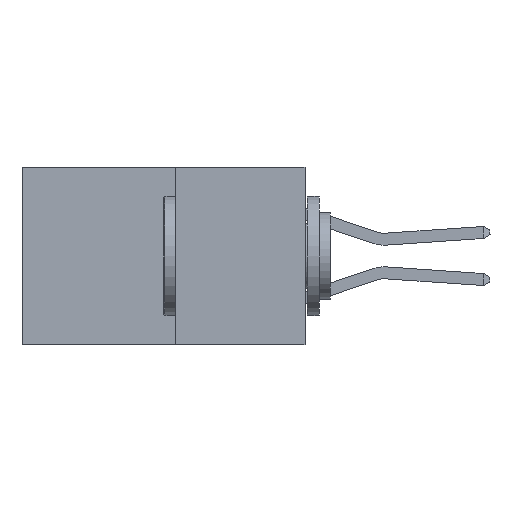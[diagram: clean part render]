
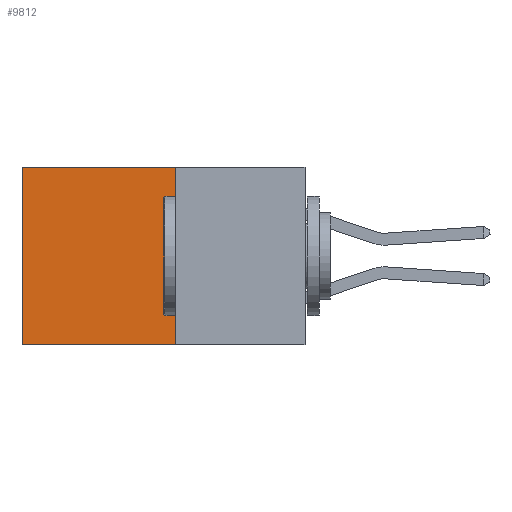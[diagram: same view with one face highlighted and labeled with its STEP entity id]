
A CAD part, left-side view. The second image highlights one B-rep face of the part: STEP entity #9812.
In plain terms, the highlighted planar face has unit normal (-1, 0, 0).
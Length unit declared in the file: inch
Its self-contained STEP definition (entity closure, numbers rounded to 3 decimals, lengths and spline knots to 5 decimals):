
#578 = EDGE_CURVE ( 'NONE', #14383, #9745, #9992, .T. ) ;
#730 = DIRECTION ( 'NONE',  ( 0., 0., -1. ) ) ;
#804 = DIRECTION ( 'NONE',  ( 0., 1., 0. ) ) ;
#988 = CARTESIAN_POINT ( 'NONE',  ( 0.277, 0.27, -0.37 ) ) ;
#1501 = VECTOR ( 'NONE', #804, 39.37008 ) ;
#1978 = CARTESIAN_POINT ( 'NONE',  ( 0.277, 0.59, -0.37 ) ) ;
#2117 = LINE ( 'NONE', #7203, #9323 ) ;
#2404 = ORIENTED_EDGE ( 'NONE', *, *, #6693, .T. ) ;
#3369 = AXIS2_PLACEMENT_3D ( 'NONE', #15497, #8849, #730 ) ;
#3455 = CARTESIAN_POINT ( 'NONE',  ( 0.277, 0.27, -0.37 ) ) ;
#4028 = CARTESIAN_POINT ( 'NONE',  ( 0.277, 0.27, 0. ) ) ;
#4515 = FACE_OUTER_BOUND ( 'NONE', #9833, .T. ) ;
#5127 = LINE ( 'NONE', #3455, #1501 ) ;
#6520 = DIRECTION ( 'NONE',  ( 0., 0., -1. ) ) ;
#6643 = ORIENTED_EDGE ( 'NONE', *, *, #15002, .F. ) ;
#6693 = EDGE_CURVE ( 'NONE', #9190, #14383, #2117, .T. ) ;
#6976 = DIRECTION ( 'NONE',  ( 0., 1., 0. ) ) ;
#6990 = VECTOR ( 'NONE', #6520, 39.37008 ) ;
#7203 = CARTESIAN_POINT ( 'NONE',  ( 0.277, 0.27, 0. ) ) ;
#7658 = CARTESIAN_POINT ( 'NONE',  ( 0.277, 0.59, -0.37 ) ) ;
#8849 = DIRECTION ( 'NONE',  ( 1., 0., 0. ) ) ;
#8980 = DIRECTION ( 'NONE',  ( 0., 0., -1. ) ) ;
#9078 = CARTESIAN_POINT ( 'NONE',  ( 0.277, 0.59, 0. ) ) ;
#9190 = VERTEX_POINT ( 'NONE', #4028 ) ;
#9323 = VECTOR ( 'NONE', #6976, 39.37008 ) ;
#9745 = VERTEX_POINT ( 'NONE', #1978 ) ;
#9812 = ADVANCED_FACE ( 'NONE', ( #4515 ), #12782, .F. ) ;
#9833 = EDGE_LOOP ( 'NONE', ( #14343, #16789, #6643, #2404 ) ) ;
#9992 = LINE ( 'NONE', #7658, #10405 ) ;
#10405 = VECTOR ( 'NONE', #8980, 39.37008 ) ;
#10542 = LINE ( 'NONE', #12874, #6990 ) ;
#11164 = VERTEX_POINT ( 'NONE', #988 ) ;
#12782 = PLANE ( 'NONE',  #3369 ) ;
#12874 = CARTESIAN_POINT ( 'NONE',  ( 0.277, 0.27, -0.37 ) ) ;
#13529 = EDGE_CURVE ( 'NONE', #11164, #9745, #5127, .T. ) ;
#14343 = ORIENTED_EDGE ( 'NONE', *, *, #578, .T. ) ;
#14383 = VERTEX_POINT ( 'NONE', #9078 ) ;
#15002 = EDGE_CURVE ( 'NONE', #9190, #11164, #10542, .T. ) ;
#15497 = CARTESIAN_POINT ( 'NONE',  ( 0.277, 0.27, -0.37 ) ) ;
#16789 = ORIENTED_EDGE ( 'NONE', *, *, #13529, .F. ) ;
